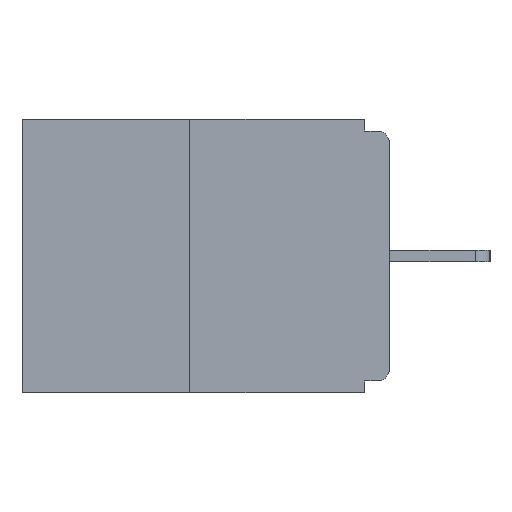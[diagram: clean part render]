
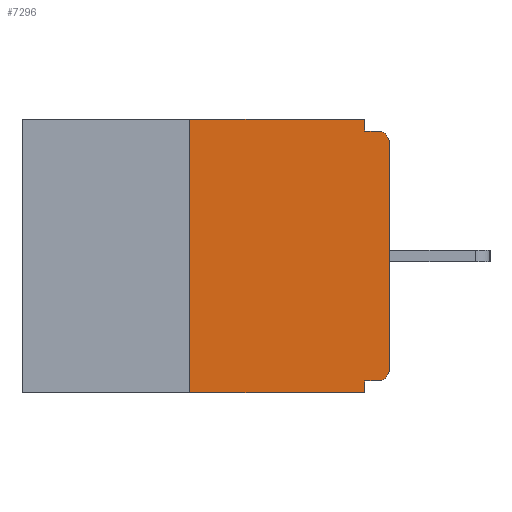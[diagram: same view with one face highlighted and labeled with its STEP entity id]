
A CAD part, left-side view. The second image highlights one B-rep face of the part: STEP entity #7296.
In plain terms, the highlighted planar face has unit normal (-1, 0, 0).
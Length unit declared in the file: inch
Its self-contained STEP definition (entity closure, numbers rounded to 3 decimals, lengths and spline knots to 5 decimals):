
#534 = EDGE_CURVE ( 'NONE', #12552, #19336, #19805, .T. ) ;
#937 = DIRECTION ( 'NONE',  ( 0., 0., -1. ) ) ;
#1409 = LINE ( 'NONE', #9428, #12227 ) ;
#1707 = DIRECTION ( 'NONE',  ( 0., 0., 1. ) ) ;
#1799 = CARTESIAN_POINT ( 'NONE',  ( 0., 0.031, -0.015 ) ) ;
#2121 = EDGE_CURVE ( 'NONE', #18071, #14114, #18764, .T. ) ;
#2700 = VECTOR ( 'NONE', #7128, 39.37008 ) ;
#5100 = EDGE_CURVE ( 'NONE', #8526, #14114, #14675, .T. ) ;
#5153 = CARTESIAN_POINT ( 'NONE',  ( 0., 0., -0.015 ) ) ;
#5289 = DIRECTION ( 'NONE',  ( 0., -1., 0. ) ) ;
#5323 = DIRECTION ( 'NONE',  ( 0., -1., 0. ) ) ;
#5631 = CARTESIAN_POINT ( 'NONE',  ( 0., 0.031, -0.343 ) ) ;
#5714 = DIRECTION ( 'NONE',  ( 0., 0., 1. ) ) ;
#5974 = CARTESIAN_POINT ( 'NONE',  ( 0., 0.015, -0.03 ) ) ;
#6208 = DIRECTION ( 'NONE',  ( -1., 0., 0. ) ) ;
#6319 = CARTESIAN_POINT ( 'NONE',  ( 0., 0.46, 0. ) ) ;
#6360 = CARTESIAN_POINT ( 'NONE',  ( 0., 0.015, -0.015 ) ) ;
#6533 = LINE ( 'NONE', #14534, #19673 ) ;
#7128 = DIRECTION ( 'NONE',  ( 0., -1., 0. ) ) ;
#7250 = LINE ( 'NONE', #20784, #2700 ) ;
#7289 = CARTESIAN_POINT ( 'NONE',  ( 0., 0.031, 0. ) ) ;
#7296 = ADVANCED_FACE ( 'NONE', ( #10531 ), #21715, .F. ) ;
#8343 = AXIS2_PLACEMENT_3D ( 'NONE', #6319, #20047, #11569 ) ;
#8526 = VERTEX_POINT ( 'NONE', #18409 ) ;
#9080 = CARTESIAN_POINT ( 'NONE',  ( 0., 0.031, -0.343 ) ) ;
#9167 = ORIENTED_EDGE ( 'NONE', *, *, #2121, .T. ) ;
#9372 = VERTEX_POINT ( 'NONE', #9380 ) ;
#9380 = CARTESIAN_POINT ( 'NONE',  ( 0., 0., -0.03 ) ) ;
#9428 = CARTESIAN_POINT ( 'NONE',  ( 0., 0.031, 0. ) ) ;
#9486 = ORIENTED_EDGE ( 'NONE', *, *, #21011, .T. ) ;
#9874 = EDGE_CURVE ( 'NONE', #17450, #8526, #6533, .T. ) ;
#9935 = ORIENTED_EDGE ( 'NONE', *, *, #20410, .F. ) ;
#10531 = FACE_OUTER_BOUND ( 'NONE', #12373, .T. ) ;
#10676 = VECTOR ( 'NONE', #5289, 39.37008 ) ;
#10690 = CARTESIAN_POINT ( 'NONE',  ( 0., 0.46, -0.343 ) ) ;
#10813 = EDGE_CURVE ( 'NONE', #20470, #12552, #1409, .T. ) ;
#11569 = DIRECTION ( 'NONE',  ( 0., 0., -1. ) ) ;
#11979 = CARTESIAN_POINT ( 'NONE',  ( 0., 0.25, 0. ) ) ;
#12099 = AXIS2_PLACEMENT_3D ( 'NONE', #19696, #6208, #937 ) ;
#12227 = VECTOR ( 'NONE', #17685, 39.37008 ) ;
#12373 = EDGE_LOOP ( 'NONE', ( #9935, #17559, #9167, #16575, #20649, #9486, #22251, #13240, #17414, #19538 ) ) ;
#12552 = VERTEX_POINT ( 'NONE', #1799 ) ;
#12585 = CARTESIAN_POINT ( 'NONE',  ( 0., 0., -0.313 ) ) ;
#13240 = ORIENTED_EDGE ( 'NONE', *, *, #16528, .T. ) ;
#13400 = CIRCLE ( 'NONE', #18354, 0.015 ) ;
#13997 = CARTESIAN_POINT ( 'NONE',  ( 0., 0.015, -0.328 ) ) ;
#14114 = VERTEX_POINT ( 'NONE', #5631 ) ;
#14534 = CARTESIAN_POINT ( 'NONE',  ( 0., 0., -0.328 ) ) ;
#14675 = LINE ( 'NONE', #9080, #20038 ) ;
#15847 = LINE ( 'NONE', #11979, #19118 ) ;
#16231 = CARTESIAN_POINT ( 'NONE',  ( 0., 0.25, 0. ) ) ;
#16253 = DIRECTION ( 'NONE',  ( 0., 0., -1. ) ) ;
#16308 = VECTOR ( 'NONE', #5323, 39.37008 ) ;
#16528 = EDGE_CURVE ( 'NONE', #9372, #19336, #13400, .T. ) ;
#16575 = ORIENTED_EDGE ( 'NONE', *, *, #5100, .F. ) ;
#17414 = ORIENTED_EDGE ( 'NONE', *, *, #534, .F. ) ;
#17450 = VERTEX_POINT ( 'NONE', #13997 ) ;
#17559 = ORIENTED_EDGE ( 'NONE', *, *, #21583, .F. ) ;
#17610 = VERTEX_POINT ( 'NONE', #12585 ) ;
#17685 = DIRECTION ( 'NONE',  ( 0., 0., -1. ) ) ;
#17734 = VERTEX_POINT ( 'NONE', #16231 ) ;
#17782 = CARTESIAN_POINT ( 'NONE',  ( 0., 0., 0. ) ) ;
#17984 = DIRECTION ( 'NONE',  ( 0., 0., -1. ) ) ;
#18071 = VERTEX_POINT ( 'NONE', #20430 ) ;
#18341 = EDGE_CURVE ( 'NONE', #17610, #9372, #19541, .T. ) ;
#18354 = AXIS2_PLACEMENT_3D ( 'NONE', #5974, #19688, #17984 ) ;
#18409 = CARTESIAN_POINT ( 'NONE',  ( 0., 0.031, -0.328 ) ) ;
#18482 = VECTOR ( 'NONE', #5714, 39.37008 ) ;
#18620 = CIRCLE ( 'NONE', #12099, 0.015 ) ;
#18764 = LINE ( 'NONE', #10690, #16308 ) ;
#19118 = VECTOR ( 'NONE', #1707, 39.37008 ) ;
#19336 = VERTEX_POINT ( 'NONE', #6360 ) ;
#19538 = ORIENTED_EDGE ( 'NONE', *, *, #10813, .F. ) ;
#19541 = LINE ( 'NONE', #17782, #18482 ) ;
#19673 = VECTOR ( 'NONE', #21294, 39.37008 ) ;
#19688 = DIRECTION ( 'NONE',  ( -1., 0., 0. ) ) ;
#19696 = CARTESIAN_POINT ( 'NONE',  ( 0., 0.015, -0.313 ) ) ;
#19805 = LINE ( 'NONE', #5153, #10676 ) ;
#20038 = VECTOR ( 'NONE', #16253, 39.37008 ) ;
#20047 = DIRECTION ( 'NONE',  ( 1., 0., 0. ) ) ;
#20410 = EDGE_CURVE ( 'NONE', #17734, #20470, #7250, .T. ) ;
#20430 = CARTESIAN_POINT ( 'NONE',  ( 0., 0.25, -0.343 ) ) ;
#20470 = VERTEX_POINT ( 'NONE', #7289 ) ;
#20649 = ORIENTED_EDGE ( 'NONE', *, *, #9874, .F. ) ;
#20784 = CARTESIAN_POINT ( 'NONE',  ( 0., 0.46, 0. ) ) ;
#21011 = EDGE_CURVE ( 'NONE', #17450, #17610, #18620, .T. ) ;
#21294 = DIRECTION ( 'NONE',  ( 0., 1., 0. ) ) ;
#21583 = EDGE_CURVE ( 'NONE', #18071, #17734, #15847, .T. ) ;
#21715 = PLANE ( 'NONE',  #8343 ) ;
#22251 = ORIENTED_EDGE ( 'NONE', *, *, #18341, .T. ) ;
